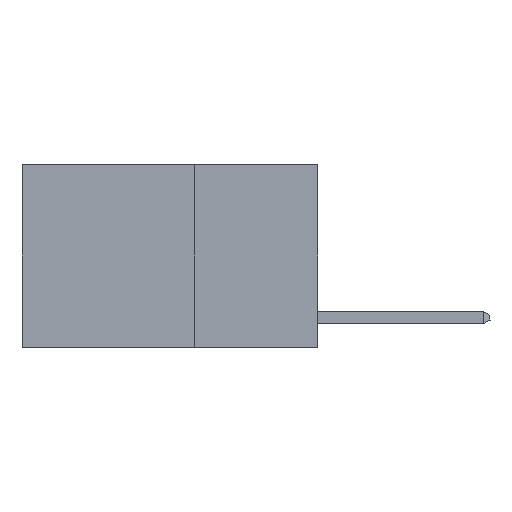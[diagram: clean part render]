
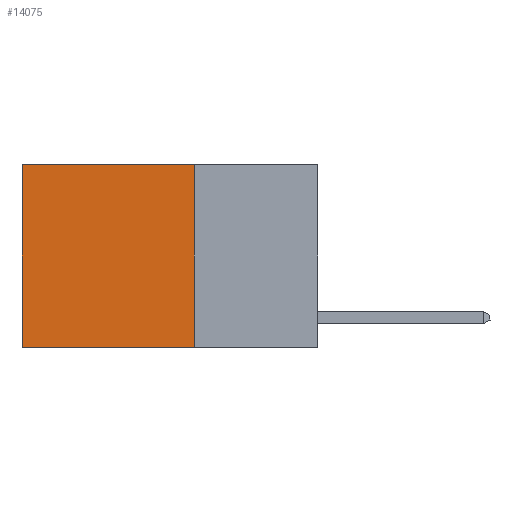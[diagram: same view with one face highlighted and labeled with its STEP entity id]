
A CAD part, left-side view. The second image highlights one B-rep face of the part: STEP entity #14075.
In plain terms, the highlighted planar face has unit normal (-1, 0, 0).
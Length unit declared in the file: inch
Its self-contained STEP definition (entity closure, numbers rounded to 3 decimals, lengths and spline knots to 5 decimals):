
#103 = CARTESIAN_POINT ( 'NONE',  ( 0.2625, 0.25, 0. ) ) ;
#915 = LINE ( 'NONE', #103, #14407 ) ;
#1305 = CARTESIAN_POINT ( 'NONE',  ( 0.2625, 0.6, 0. ) ) ;
#1445 = LINE ( 'NONE', #10721, #14900 ) ;
#1892 = FACE_OUTER_BOUND ( 'NONE', #2382, .T. ) ;
#2056 = EDGE_CURVE ( 'NONE', #7155, #14694, #7016, .T. ) ;
#2319 = AXIS2_PLACEMENT_3D ( 'NONE', #12504, #4770, #13818 ) ;
#2382 = EDGE_LOOP ( 'NONE', ( #13051, #16844, #3557, #6980 ) ) ;
#3557 = ORIENTED_EDGE ( 'NONE', *, *, #16271, .F. ) ;
#3594 = VECTOR ( 'NONE', #7564, 39.37008 ) ;
#4270 = DIRECTION ( 'NONE',  ( 0., 0., -1. ) ) ;
#4770 = DIRECTION ( 'NONE',  ( 1., 0., 0. ) ) ;
#5227 = DIRECTION ( 'NONE',  ( 0., 0., -1. ) ) ;
#6635 = CARTESIAN_POINT ( 'NONE',  ( 0.2625, 0.25, -0.37 ) ) ;
#6688 = DIRECTION ( 'NONE',  ( 0., 1., 0. ) ) ;
#6980 = ORIENTED_EDGE ( 'NONE', *, *, #11313, .T. ) ;
#7016 = LINE ( 'NONE', #9068, #3594 ) ;
#7155 = VERTEX_POINT ( 'NONE', #6635 ) ;
#7169 = CARTESIAN_POINT ( 'NONE',  ( 0.2625, 0.6, -0.37 ) ) ;
#7564 = DIRECTION ( 'NONE',  ( 0., 1., 0. ) ) ;
#9068 = CARTESIAN_POINT ( 'NONE',  ( 0.2625, 0.25, -0.37 ) ) ;
#10406 = CARTESIAN_POINT ( 'NONE',  ( 0.2625, 0.6, 0. ) ) ;
#10721 = CARTESIAN_POINT ( 'NONE',  ( 0.2625, 0.25, 0. ) ) ;
#11221 = PLANE ( 'NONE',  #2319 ) ;
#11313 = EDGE_CURVE ( 'NONE', #11916, #16165, #915, .T. ) ;
#11916 = VERTEX_POINT ( 'NONE', #14315 ) ;
#11918 = VECTOR ( 'NONE', #5227, 39.37008 ) ;
#12504 = CARTESIAN_POINT ( 'NONE',  ( 0.2625, 0.25, 0. ) ) ;
#13051 = ORIENTED_EDGE ( 'NONE', *, *, #14994, .T. ) ;
#13818 = DIRECTION ( 'NONE',  ( 0., 0., -1. ) ) ;
#14075 = ADVANCED_FACE ( 'NONE', ( #1892 ), #11221, .F. ) ;
#14315 = CARTESIAN_POINT ( 'NONE',  ( 0.2625, 0.25, 0. ) ) ;
#14407 = VECTOR ( 'NONE', #6688, 39.37008 ) ;
#14694 = VERTEX_POINT ( 'NONE', #7169 ) ;
#14900 = VECTOR ( 'NONE', #4270, 39.37008 ) ;
#14994 = EDGE_CURVE ( 'NONE', #16165, #14694, #15327, .T. ) ;
#15327 = LINE ( 'NONE', #10406, #11918 ) ;
#16165 = VERTEX_POINT ( 'NONE', #1305 ) ;
#16271 = EDGE_CURVE ( 'NONE', #11916, #7155, #1445, .T. ) ;
#16844 = ORIENTED_EDGE ( 'NONE', *, *, #2056, .F. ) ;
